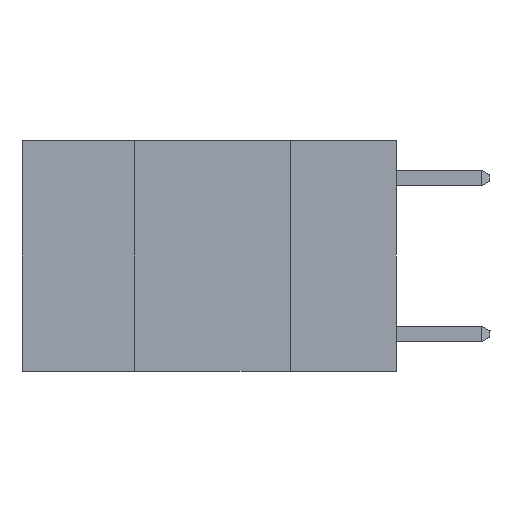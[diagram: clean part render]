
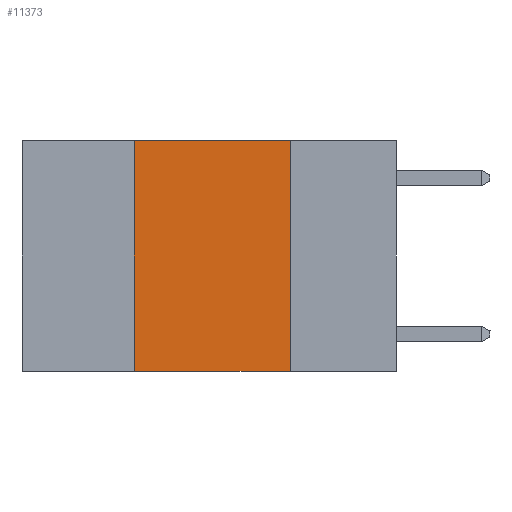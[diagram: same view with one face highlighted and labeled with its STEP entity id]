
A CAD part, left-side view. The second image highlights one B-rep face of the part: STEP entity #11373.
In plain terms, the highlighted planar face has unit normal (-1, 0, 0).
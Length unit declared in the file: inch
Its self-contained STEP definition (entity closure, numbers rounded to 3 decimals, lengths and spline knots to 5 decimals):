
#178 = CARTESIAN_POINT ( 'NONE',  ( 0., 0.17, 0. ) ) ;
#513 = VERTEX_POINT ( 'NONE', #15872 ) ;
#3358 = ORIENTED_EDGE ( 'NONE', *, *, #14276, .T. ) ;
#3585 = ORIENTED_EDGE ( 'NONE', *, *, #20430, .F. ) ;
#6193 = DIRECTION ( 'NONE',  ( 0., 0., 1. ) ) ;
#6725 = CARTESIAN_POINT ( 'NONE',  ( 0., 0.6, 0. ) ) ;
#7070 = ORIENTED_EDGE ( 'NONE', *, *, #23865, .F. ) ;
#7098 = ORIENTED_EDGE ( 'NONE', *, *, #10245, .F. ) ;
#8153 = CARTESIAN_POINT ( 'NONE',  ( 0., 0.6, -0.37 ) ) ;
#9243 = DIRECTION ( 'NONE',  ( 0., -1., 0. ) ) ;
#10245 = EDGE_CURVE ( 'NONE', #16894, #21038, #20569, .T. ) ;
#10831 = PLANE ( 'NONE',  #24946 ) ;
#10935 = VECTOR ( 'NONE', #25348, 39.37008 ) ;
#11373 = ADVANCED_FACE ( 'NONE', ( #22383 ), #10831, .F. ) ;
#12236 = CARTESIAN_POINT ( 'NONE',  ( 0., 0.42, 0. ) ) ;
#14048 = VECTOR ( 'NONE', #9243, 39.37008 ) ;
#14276 = EDGE_CURVE ( 'NONE', #513, #14500, #20690, .T. ) ;
#14500 = VERTEX_POINT ( 'NONE', #16841 ) ;
#15781 = DIRECTION ( 'NONE',  ( 0., 0., -1. ) ) ;
#15872 = CARTESIAN_POINT ( 'NONE',  ( 0., 0.42, -0.37 ) ) ;
#16841 = CARTESIAN_POINT ( 'NONE',  ( 0., 0.17, -0.37 ) ) ;
#16894 = VERTEX_POINT ( 'NONE', #12236 ) ;
#16983 = EDGE_LOOP ( 'NONE', ( #3585, #7098, #7070, #3358 ) ) ;
#20430 = EDGE_CURVE ( 'NONE', #21038, #14500, #24710, .T. ) ;
#20569 = LINE ( 'NONE', #6725, #14048 ) ;
#20690 = LINE ( 'NONE', #8153, #27106 ) ;
#20694 = VECTOR ( 'NONE', #6193, 39.37008 ) ;
#21038 = VERTEX_POINT ( 'NONE', #178 ) ;
#22383 = FACE_OUTER_BOUND ( 'NONE', #16983, .T. ) ;
#23865 = EDGE_CURVE ( 'NONE', #513, #16894, #27846, .T. ) ;
#24710 = LINE ( 'NONE', #27665, #10935 ) ;
#24946 = AXIS2_PLACEMENT_3D ( 'NONE', #27871, #30241, #15781 ) ;
#25343 = DIRECTION ( 'NONE',  ( 0., -1., 0. ) ) ;
#25348 = DIRECTION ( 'NONE',  ( 0., 0., -1. ) ) ;
#27106 = VECTOR ( 'NONE', #25343, 39.37008 ) ;
#27665 = CARTESIAN_POINT ( 'NONE',  ( 0., 0.17, 0. ) ) ;
#27846 = LINE ( 'NONE', #30522, #20694 ) ;
#27871 = CARTESIAN_POINT ( 'NONE',  ( 0., 0.6, 0. ) ) ;
#30241 = DIRECTION ( 'NONE',  ( 1., 0., 0. ) ) ;
#30522 = CARTESIAN_POINT ( 'NONE',  ( 0., 0.42, 0. ) ) ;
